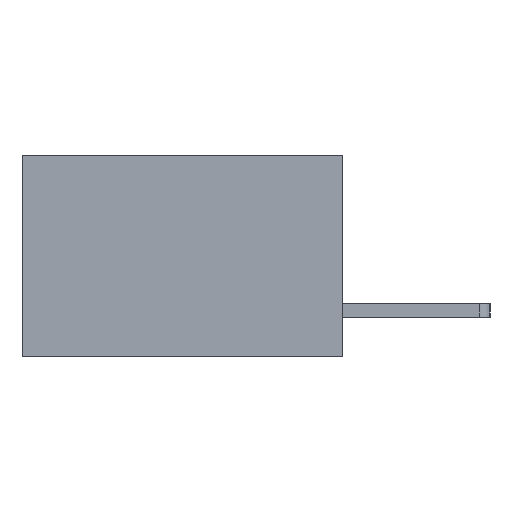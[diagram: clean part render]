
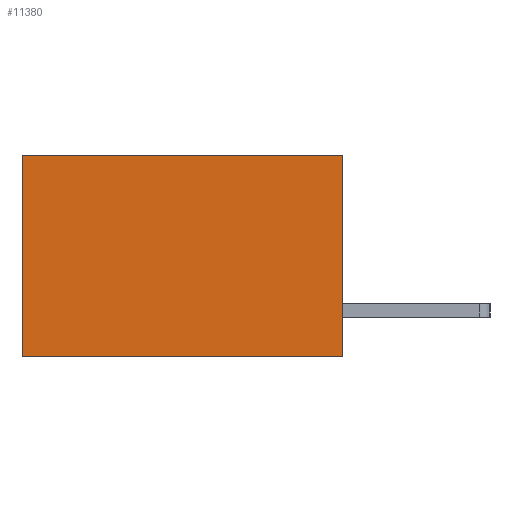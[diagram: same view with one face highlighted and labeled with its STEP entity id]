
A CAD part, left-side view. The second image highlights one B-rep face of the part: STEP entity #11380.
In plain terms, the highlighted planar face has unit normal (-1, 0, 0).
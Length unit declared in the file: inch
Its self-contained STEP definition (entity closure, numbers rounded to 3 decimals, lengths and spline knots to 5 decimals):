
#703 = CARTESIAN_POINT ( 'NONE',  ( 0.277, 0.59, -0.37 ) ) ;
#832 = VERTEX_POINT ( 'NONE', #12209 ) ;
#944 = VERTEX_POINT ( 'NONE', #703 ) ;
#1423 = VERTEX_POINT ( 'NONE', #2706 ) ;
#1567 = LINE ( 'NONE', #1635, #3987 ) ;
#1635 = CARTESIAN_POINT ( 'NONE',  ( 0.277, 0., 0. ) ) ;
#2706 = CARTESIAN_POINT ( 'NONE',  ( 0.277, 0., 0. ) ) ;
#2783 = CARTESIAN_POINT ( 'NONE',  ( 0.277, 0., -0.37 ) ) ;
#3067 = AXIS2_PLACEMENT_3D ( 'NONE', #5204, #12232, #6179 ) ;
#3448 = VECTOR ( 'NONE', #6848, 39.37008 ) ;
#3501 = VECTOR ( 'NONE', #7665, 39.37008 ) ;
#3819 = DIRECTION ( 'NONE',  ( 0., 1., 0. ) ) ;
#3987 = VECTOR ( 'NONE', #8852, 39.37008 ) ;
#5204 = CARTESIAN_POINT ( 'NONE',  ( 0.277, 0., -0.37 ) ) ;
#5592 = CARTESIAN_POINT ( 'NONE',  ( 0.277, 0., -0.37 ) ) ;
#5891 = EDGE_CURVE ( 'NONE', #832, #944, #6479, .T. ) ;
#6119 = LINE ( 'NONE', #6450, #3448 ) ;
#6179 = DIRECTION ( 'NONE',  ( 0., 0., -1. ) ) ;
#6450 = CARTESIAN_POINT ( 'NONE',  ( 0.277, 0., -0.37 ) ) ;
#6479 = LINE ( 'NONE', #7639, #3501 ) ;
#6548 = FACE_OUTER_BOUND ( 'NONE', #12358, .T. ) ;
#6848 = DIRECTION ( 'NONE',  ( 0., 0., -1. ) ) ;
#7031 = VECTOR ( 'NONE', #3819, 39.37008 ) ;
#7434 = ORIENTED_EDGE ( 'NONE', *, *, #12818, .T. ) ;
#7639 = CARTESIAN_POINT ( 'NONE',  ( 0.277, 0.59, -0.37 ) ) ;
#7665 = DIRECTION ( 'NONE',  ( 0., 0., -1. ) ) ;
#7769 = EDGE_CURVE ( 'NONE', #1423, #7828, #6119, .T. ) ;
#7828 = VERTEX_POINT ( 'NONE', #5592 ) ;
#8049 = ORIENTED_EDGE ( 'NONE', *, *, #11159, .F. ) ;
#8061 = ORIENTED_EDGE ( 'NONE', *, *, #7769, .F. ) ;
#8236 = PLANE ( 'NONE',  #3067 ) ;
#8269 = ORIENTED_EDGE ( 'NONE', *, *, #5891, .T. ) ;
#8852 = DIRECTION ( 'NONE',  ( 0., 1., 0. ) ) ;
#9509 = LINE ( 'NONE', #2783, #7031 ) ;
#11159 = EDGE_CURVE ( 'NONE', #7828, #944, #9509, .T. ) ;
#11380 = ADVANCED_FACE ( 'NONE', ( #6548 ), #8236, .F. ) ;
#12209 = CARTESIAN_POINT ( 'NONE',  ( 0.277, 0.59, 0. ) ) ;
#12232 = DIRECTION ( 'NONE',  ( 1., 0., 0. ) ) ;
#12358 = EDGE_LOOP ( 'NONE', ( #8269, #8049, #8061, #7434 ) ) ;
#12818 = EDGE_CURVE ( 'NONE', #1423, #832, #1567, .T. ) ;
